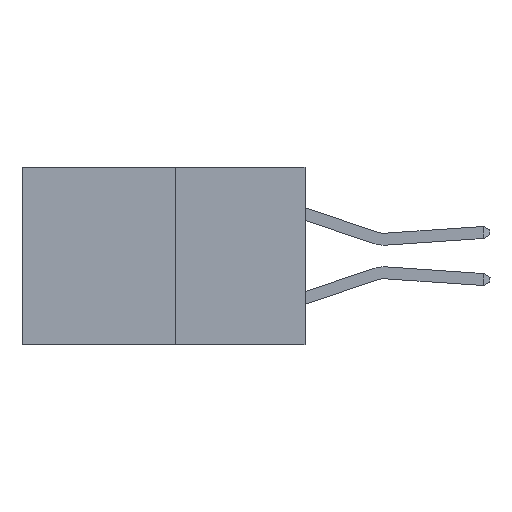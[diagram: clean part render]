
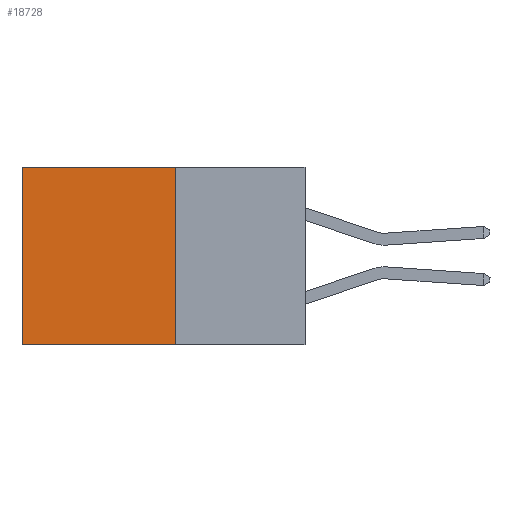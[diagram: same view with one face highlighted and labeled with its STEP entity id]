
A CAD part, left-side view. The second image highlights one B-rep face of the part: STEP entity #18728.
In plain terms, the highlighted planar face has unit normal (-1, 0, 0).
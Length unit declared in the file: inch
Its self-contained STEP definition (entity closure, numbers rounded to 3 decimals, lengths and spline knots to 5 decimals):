
#339 = EDGE_LOOP ( 'NONE', ( #7609, #20012, #26234, #14768 ) ) ;
#417 = VECTOR ( 'NONE', #21623, 39.37008 ) ;
#1653 = AXIS2_PLACEMENT_3D ( 'NONE', #16162, #23291, #9002 ) ;
#1887 = FACE_OUTER_BOUND ( 'NONE', #339, .T. ) ;
#2023 = EDGE_CURVE ( 'NONE', #5044, #7254, #24144, .T. ) ;
#2168 = EDGE_CURVE ( 'NONE', #9274, #16585, #24732, .T. ) ;
#3803 = CARTESIAN_POINT ( 'NONE',  ( 0.277, 0.27, -0.37 ) ) ;
#4007 = DIRECTION ( 'NONE',  ( 0., 0., -1. ) ) ;
#4524 = CARTESIAN_POINT ( 'NONE',  ( 0.277, 0.59, -0.37 ) ) ;
#5044 = VERTEX_POINT ( 'NONE', #6660 ) ;
#6660 = CARTESIAN_POINT ( 'NONE',  ( 0.277, 0.59, 0. ) ) ;
#7254 = VERTEX_POINT ( 'NONE', #4524 ) ;
#7609 = ORIENTED_EDGE ( 'NONE', *, *, #2023, .T. ) ;
#8203 = EDGE_CURVE ( 'NONE', #9274, #5044, #19618, .T. ) ;
#8938 = DIRECTION ( 'NONE',  ( 0., 0., -1. ) ) ;
#9002 = DIRECTION ( 'NONE',  ( 0., 0., -1. ) ) ;
#9274 = VERTEX_POINT ( 'NONE', #18499 ) ;
#11482 = VECTOR ( 'NONE', #8938, 39.37008 ) ;
#11622 = CARTESIAN_POINT ( 'NONE',  ( 0.277, 0.27, -0.37 ) ) ;
#12606 = CARTESIAN_POINT ( 'NONE',  ( 0.277, 0.59, -0.37 ) ) ;
#14768 = ORIENTED_EDGE ( 'NONE', *, *, #8203, .T. ) ;
#16162 = CARTESIAN_POINT ( 'NONE',  ( 0.277, 0.27, -0.37 ) ) ;
#16585 = VERTEX_POINT ( 'NONE', #28789 ) ;
#17114 = EDGE_CURVE ( 'NONE', #16585, #7254, #29140, .T. ) ;
#18499 = CARTESIAN_POINT ( 'NONE',  ( 0.277, 0.27, 0. ) ) ;
#18728 = ADVANCED_FACE ( 'NONE', ( #1887 ), #20949, .F. ) ;
#19232 = VECTOR ( 'NONE', #4007, 39.37008 ) ;
#19263 = CARTESIAN_POINT ( 'NONE',  ( 0.277, 0.27, 0. ) ) ;
#19618 = LINE ( 'NONE', #19263, #417 ) ;
#20012 = ORIENTED_EDGE ( 'NONE', *, *, #17114, .F. ) ;
#20778 = VECTOR ( 'NONE', #23602, 39.37008 ) ;
#20949 = PLANE ( 'NONE',  #1653 ) ;
#21623 = DIRECTION ( 'NONE',  ( 0., 1., 0. ) ) ;
#23291 = DIRECTION ( 'NONE',  ( 1., 0., 0. ) ) ;
#23602 = DIRECTION ( 'NONE',  ( 0., 1., 0. ) ) ;
#24144 = LINE ( 'NONE', #12606, #11482 ) ;
#24732 = LINE ( 'NONE', #3803, #19232 ) ;
#26234 = ORIENTED_EDGE ( 'NONE', *, *, #2168, .F. ) ;
#28789 = CARTESIAN_POINT ( 'NONE',  ( 0.277, 0.27, -0.37 ) ) ;
#29140 = LINE ( 'NONE', #11622, #20778 ) ;
